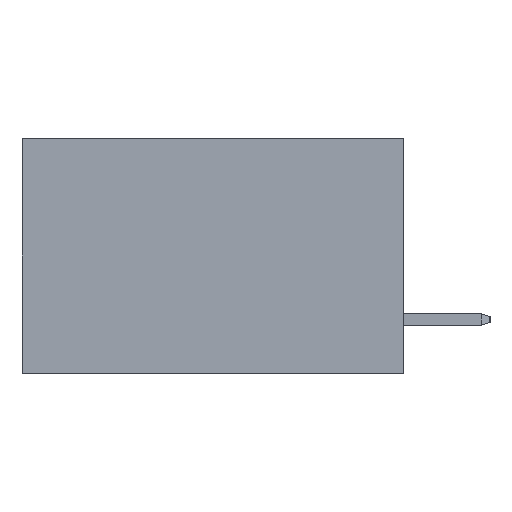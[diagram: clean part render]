
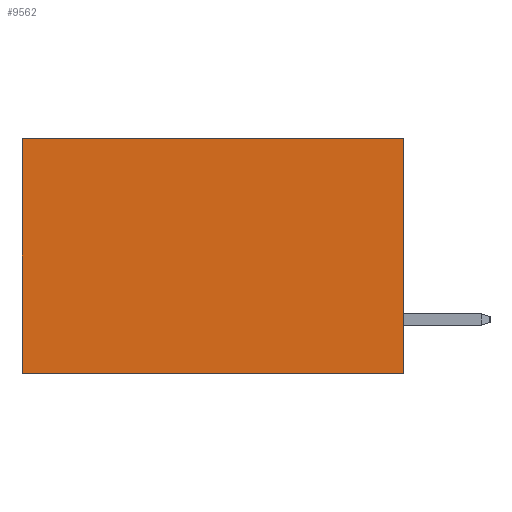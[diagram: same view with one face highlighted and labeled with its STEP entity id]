
A CAD part, left-side view. The second image highlights one B-rep face of the part: STEP entity #9562.
In plain terms, the highlighted planar face has unit normal (-1, 0, 0).
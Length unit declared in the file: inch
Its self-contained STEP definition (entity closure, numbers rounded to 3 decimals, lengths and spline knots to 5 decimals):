
#468 = VECTOR ( 'NONE', #4780, 39.37008 ) ;
#729 = VERTEX_POINT ( 'NONE', #3894 ) ;
#1218 = CARTESIAN_POINT ( 'NONE',  ( 0.2875, 0.6, 0. ) ) ;
#2689 = LINE ( 'NONE', #9731, #9836 ) ;
#3300 = CARTESIAN_POINT ( 'NONE',  ( 0.2875, 0.6, 0. ) ) ;
#3371 = EDGE_CURVE ( 'NONE', #8524, #8827, #6612, .T. ) ;
#3421 = DIRECTION ( 'NONE',  ( 0., 0., -1. ) ) ;
#3439 = LINE ( 'NONE', #3300, #3783 ) ;
#3770 = EDGE_LOOP ( 'NONE', ( #7504, #13471, #4452, #11242 ) ) ;
#3783 = VECTOR ( 'NONE', #9680, 39.37008 ) ;
#3894 = CARTESIAN_POINT ( 'NONE',  ( 0.2875, 0.6, -0.37 ) ) ;
#4452 = ORIENTED_EDGE ( 'NONE', *, *, #9505, .F. ) ;
#4780 = DIRECTION ( 'NONE',  ( 0., 1., 0. ) ) ;
#4816 = AXIS2_PLACEMENT_3D ( 'NONE', #9658, #13076, #5719 ) ;
#5719 = DIRECTION ( 'NONE',  ( 0., 0., -1. ) ) ;
#5734 = CARTESIAN_POINT ( 'NONE',  ( 0.2875, 0., -0.37 ) ) ;
#5946 = EDGE_CURVE ( 'NONE', #9333, #729, #13266, .T. ) ;
#6200 = EDGE_CURVE ( 'NONE', #8827, #729, #3439, .T. ) ;
#6612 = LINE ( 'NONE', #8491, #8944 ) ;
#7504 = ORIENTED_EDGE ( 'NONE', *, *, #6200, .T. ) ;
#7672 = PLANE ( 'NONE',  #4816 ) ;
#8491 = CARTESIAN_POINT ( 'NONE',  ( 0.2875, 0., 0. ) ) ;
#8524 = VERTEX_POINT ( 'NONE', #9745 ) ;
#8827 = VERTEX_POINT ( 'NONE', #1218 ) ;
#8944 = VECTOR ( 'NONE', #9370, 39.37008 ) ;
#9333 = VERTEX_POINT ( 'NONE', #5734 ) ;
#9370 = DIRECTION ( 'NONE',  ( 0., 1., 0. ) ) ;
#9505 = EDGE_CURVE ( 'NONE', #8524, #9333, #2689, .T. ) ;
#9562 = ADVANCED_FACE ( 'NONE', ( #11844 ), #7672, .F. ) ;
#9658 = CARTESIAN_POINT ( 'NONE',  ( 0.2875, 0., 0. ) ) ;
#9680 = DIRECTION ( 'NONE',  ( 0., 0., -1. ) ) ;
#9731 = CARTESIAN_POINT ( 'NONE',  ( 0.2875, 0., 0. ) ) ;
#9745 = CARTESIAN_POINT ( 'NONE',  ( 0.2875, 0., 0. ) ) ;
#9836 = VECTOR ( 'NONE', #3421, 39.37008 ) ;
#11149 = CARTESIAN_POINT ( 'NONE',  ( 0.2875, 0., -0.37 ) ) ;
#11242 = ORIENTED_EDGE ( 'NONE', *, *, #3371, .T. ) ;
#11844 = FACE_OUTER_BOUND ( 'NONE', #3770, .T. ) ;
#13076 = DIRECTION ( 'NONE',  ( 1., 0., 0. ) ) ;
#13266 = LINE ( 'NONE', #11149, #468 ) ;
#13471 = ORIENTED_EDGE ( 'NONE', *, *, #5946, .F. ) ;
